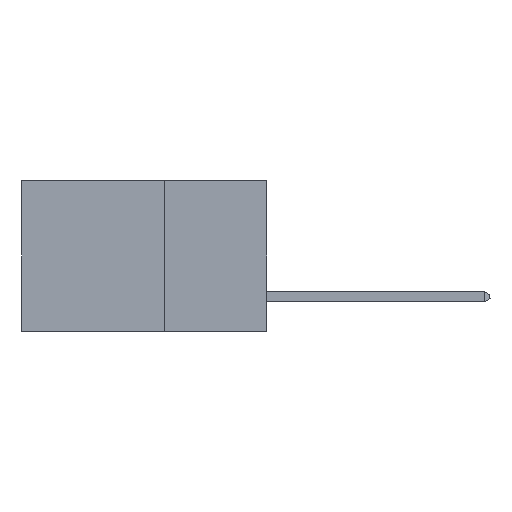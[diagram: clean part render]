
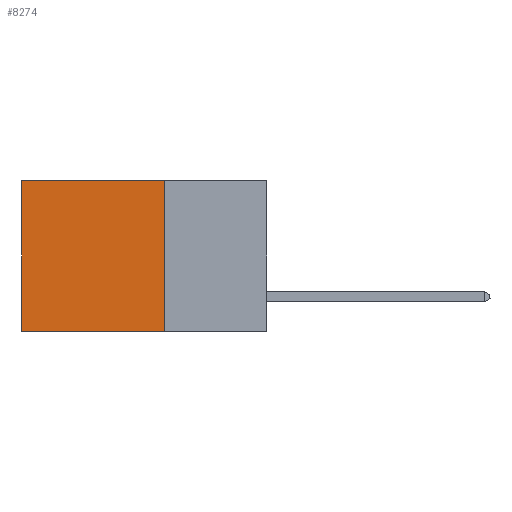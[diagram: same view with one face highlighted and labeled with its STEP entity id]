
A CAD part, left-side view. The second image highlights one B-rep face of the part: STEP entity #8274.
In plain terms, the highlighted planar face has unit normal (-1, 0, 0).
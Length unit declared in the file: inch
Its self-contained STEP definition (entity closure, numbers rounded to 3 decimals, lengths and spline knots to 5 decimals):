
#214 = CARTESIAN_POINT ( 'NONE',  ( 0.2875, 0.25, -0.37 ) ) ;
#402 = AXIS2_PLACEMENT_3D ( 'NONE', #5831, #1251, #23265 ) ;
#960 = VECTOR ( 'NONE', #15862, 39.37008 ) ;
#1251 = DIRECTION ( 'NONE',  ( 1., 0., 0. ) ) ;
#2109 = VERTEX_POINT ( 'NONE', #8897 ) ;
#3070 = VERTEX_POINT ( 'NONE', #10050 ) ;
#3473 = LINE ( 'NONE', #21276, #18175 ) ;
#4234 = EDGE_CURVE ( 'NONE', #2109, #12808, #3473, .T. ) ;
#4395 = LINE ( 'NONE', #7524, #960 ) ;
#5831 = CARTESIAN_POINT ( 'NONE',  ( 0.2875, 0.25, 0. ) ) ;
#7524 = CARTESIAN_POINT ( 'NONE',  ( 0.2875, 0.25, 0. ) ) ;
#7749 = ORIENTED_EDGE ( 'NONE', *, *, #4234, .F. ) ;
#8116 = ORIENTED_EDGE ( 'NONE', *, *, #24167, .T. ) ;
#8274 = ADVANCED_FACE ( 'NONE', ( #28323 ), #22925, .F. ) ;
#8897 = CARTESIAN_POINT ( 'NONE',  ( 0.2875, 0.25, 0. ) ) ;
#10050 = CARTESIAN_POINT ( 'NONE',  ( 0.2875, 0.6, -0.37 ) ) ;
#10698 = CARTESIAN_POINT ( 'NONE',  ( 0.2875, 0.25, -0.37 ) ) ;
#12808 = VERTEX_POINT ( 'NONE', #10698 ) ;
#15862 = DIRECTION ( 'NONE',  ( 0., 1., 0. ) ) ;
#15877 = VECTOR ( 'NONE', #19376, 39.37008 ) ;
#18112 = DIRECTION ( 'NONE',  ( 0., 0., -1. ) ) ;
#18175 = VECTOR ( 'NONE', #18112, 39.37008 ) ;
#19245 = CARTESIAN_POINT ( 'NONE',  ( 0.2875, 0.6, 0. ) ) ;
#19376 = DIRECTION ( 'NONE',  ( 0., 0., -1. ) ) ;
#20197 = VECTOR ( 'NONE', #25273, 39.37008 ) ;
#21276 = CARTESIAN_POINT ( 'NONE',  ( 0.2875, 0.25, 0. ) ) ;
#22925 = PLANE ( 'NONE',  #402 ) ;
#23265 = DIRECTION ( 'NONE',  ( 0., 0., -1. ) ) ;
#24167 = EDGE_CURVE ( 'NONE', #35545, #3070, #30655, .T. ) ;
#24372 = EDGE_LOOP ( 'NONE', ( #8116, #26769, #7749, #29783 ) ) ;
#25273 = DIRECTION ( 'NONE',  ( 0., 1., 0. ) ) ;
#26769 = ORIENTED_EDGE ( 'NONE', *, *, #33615, .F. ) ;
#27617 = LINE ( 'NONE', #214, #20197 ) ;
#28323 = FACE_OUTER_BOUND ( 'NONE', #24372, .T. ) ;
#29762 = CARTESIAN_POINT ( 'NONE',  ( 0.2875, 0.6, 0. ) ) ;
#29783 = ORIENTED_EDGE ( 'NONE', *, *, #30495, .T. ) ;
#30495 = EDGE_CURVE ( 'NONE', #2109, #35545, #4395, .T. ) ;
#30655 = LINE ( 'NONE', #19245, #15877 ) ;
#33615 = EDGE_CURVE ( 'NONE', #12808, #3070, #27617, .T. ) ;
#35545 = VERTEX_POINT ( 'NONE', #29762 ) ;
